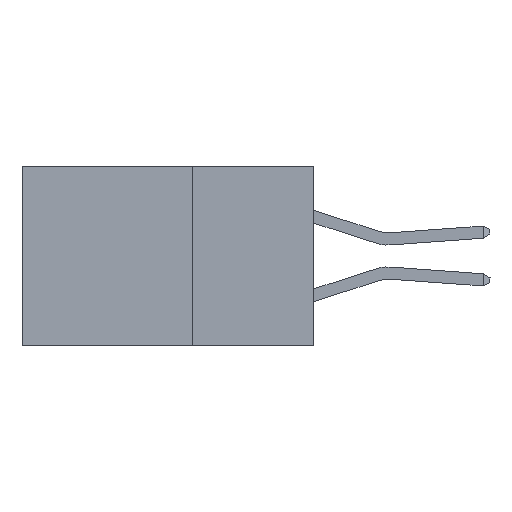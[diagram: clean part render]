
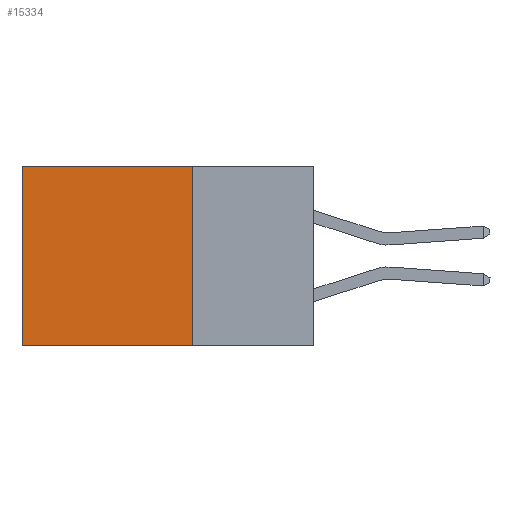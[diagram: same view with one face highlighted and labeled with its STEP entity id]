
A CAD part, left-side view. The second image highlights one B-rep face of the part: STEP entity #15334.
In plain terms, the highlighted planar face has unit normal (-1, 0, 0).
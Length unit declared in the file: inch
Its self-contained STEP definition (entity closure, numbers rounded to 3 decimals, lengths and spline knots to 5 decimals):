
#188 = VERTEX_POINT ( 'NONE', #5383 ) ;
#396 = DIRECTION ( 'NONE',  ( 0., 1., 0. ) ) ;
#479 = LINE ( 'NONE', #15103, #3734 ) ;
#829 = DIRECTION ( 'NONE',  ( 0., 1., 0. ) ) ;
#1304 = CARTESIAN_POINT ( 'NONE',  ( 0.2875, 0.25, -0.37 ) ) ;
#1326 = EDGE_LOOP ( 'NONE', ( #15761, #13705, #8164, #11582 ) ) ;
#1328 = EDGE_CURVE ( 'NONE', #188, #10618, #479, .T. ) ;
#1856 = CARTESIAN_POINT ( 'NONE',  ( 0.2875, 0.6, -0.37 ) ) ;
#2113 = VERTEX_POINT ( 'NONE', #1304 ) ;
#3734 = VECTOR ( 'NONE', #829, 39.37008 ) ;
#3844 = DIRECTION ( 'NONE',  ( 0., 0., -1. ) ) ;
#5383 = CARTESIAN_POINT ( 'NONE',  ( 0.2875, 0.25, 0. ) ) ;
#5658 = FACE_OUTER_BOUND ( 'NONE', #1326, .T. ) ;
#5850 = VECTOR ( 'NONE', #3844, 39.37008 ) ;
#6138 = CARTESIAN_POINT ( 'NONE',  ( 0.2875, 0.25, 0. ) ) ;
#6487 = CARTESIAN_POINT ( 'NONE',  ( 0.2875, 0.25, 0. ) ) ;
#7176 = VECTOR ( 'NONE', #396, 39.37008 ) ;
#7493 = DIRECTION ( 'NONE',  ( 0., 0., -1. ) ) ;
#8015 = LINE ( 'NONE', #11112, #7176 ) ;
#8045 = CARTESIAN_POINT ( 'NONE',  ( 0.2875, 0.6, 0. ) ) ;
#8164 = ORIENTED_EDGE ( 'NONE', *, *, #15532, .F. ) ;
#9340 = DIRECTION ( 'NONE',  ( 0., 0., -1. ) ) ;
#9348 = LINE ( 'NONE', #6487, #5850 ) ;
#10304 = CARTESIAN_POINT ( 'NONE',  ( 0.2875, 0.6, 0. ) ) ;
#10372 = VERTEX_POINT ( 'NONE', #1856 ) ;
#10618 = VERTEX_POINT ( 'NONE', #10304 ) ;
#11112 = CARTESIAN_POINT ( 'NONE',  ( 0.2875, 0.25, -0.37 ) ) ;
#11574 = LINE ( 'NONE', #8045, #14456 ) ;
#11582 = ORIENTED_EDGE ( 'NONE', *, *, #1328, .T. ) ;
#13452 = EDGE_CURVE ( 'NONE', #2113, #10372, #8015, .T. ) ;
#13705 = ORIENTED_EDGE ( 'NONE', *, *, #13452, .F. ) ;
#13831 = PLANE ( 'NONE',  #16788 ) ;
#14456 = VECTOR ( 'NONE', #9340, 39.37008 ) ;
#15035 = DIRECTION ( 'NONE',  ( 1., 0., 0. ) ) ;
#15103 = CARTESIAN_POINT ( 'NONE',  ( 0.2875, 0.25, 0. ) ) ;
#15334 = ADVANCED_FACE ( 'NONE', ( #5658 ), #13831, .F. ) ;
#15532 = EDGE_CURVE ( 'NONE', #188, #2113, #9348, .T. ) ;
#15761 = ORIENTED_EDGE ( 'NONE', *, *, #16294, .T. ) ;
#16294 = EDGE_CURVE ( 'NONE', #10618, #10372, #11574, .T. ) ;
#16788 = AXIS2_PLACEMENT_3D ( 'NONE', #6138, #15035, #7493 ) ;
